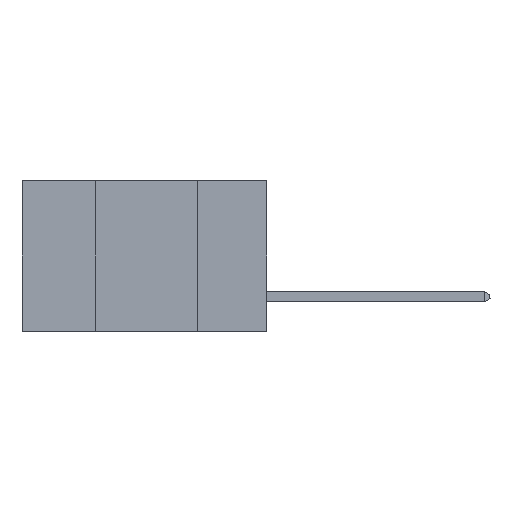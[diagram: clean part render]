
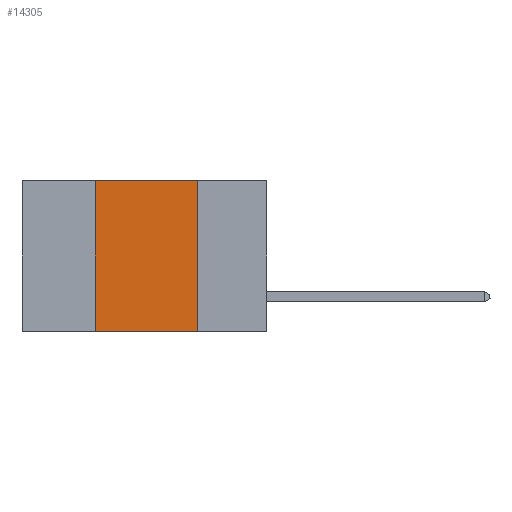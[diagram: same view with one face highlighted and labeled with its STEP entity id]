
A CAD part, left-side view. The second image highlights one B-rep face of the part: STEP entity #14305.
In plain terms, the highlighted planar face has unit normal (-1, 0, 0).
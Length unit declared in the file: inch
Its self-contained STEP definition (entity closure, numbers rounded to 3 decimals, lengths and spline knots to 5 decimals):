
#209 = VERTEX_POINT ( 'NONE', #5152 ) ;
#274 = DIRECTION ( 'NONE',  ( 0., -1., 0. ) ) ;
#516 = VECTOR ( 'NONE', #6202, 39.37008 ) ;
#661 = EDGE_CURVE ( 'NONE', #4542, #8828, #1720, .T. ) ;
#758 = CARTESIAN_POINT ( 'NONE',  ( 0., 0.6, 0. ) ) ;
#1427 = DIRECTION ( 'NONE',  ( 0., 0., 1. ) ) ;
#1720 = LINE ( 'NONE', #16820, #3463 ) ;
#3034 = VECTOR ( 'NONE', #1427, 39.37008 ) ;
#3463 = VECTOR ( 'NONE', #274, 39.37008 ) ;
#3798 = LINE ( 'NONE', #10688, #13195 ) ;
#4293 = CARTESIAN_POINT ( 'NONE',  ( 0., 0.42, 0. ) ) ;
#4542 = VERTEX_POINT ( 'NONE', #6845 ) ;
#5097 = PLANE ( 'NONE',  #12184 ) ;
#5152 = CARTESIAN_POINT ( 'NONE',  ( 0., 0.17, 0. ) ) ;
#6202 = DIRECTION ( 'NONE',  ( 0., 0., -1. ) ) ;
#6217 = EDGE_CURVE ( 'NONE', #14842, #209, #3798, .T. ) ;
#6487 = DIRECTION ( 'NONE',  ( 0., -1., 0. ) ) ;
#6845 = CARTESIAN_POINT ( 'NONE',  ( 0., 0.42, -0.37 ) ) ;
#7618 = DIRECTION ( 'NONE',  ( 1., 0., 0. ) ) ;
#7664 = FACE_OUTER_BOUND ( 'NONE', #11288, .T. ) ;
#8828 = VERTEX_POINT ( 'NONE', #13279 ) ;
#9986 = EDGE_CURVE ( 'NONE', #4542, #14842, #15908, .T. ) ;
#10352 = CARTESIAN_POINT ( 'NONE',  ( 0., 0.17, 0. ) ) ;
#10570 = ORIENTED_EDGE ( 'NONE', *, *, #9986, .F. ) ;
#10688 = CARTESIAN_POINT ( 'NONE',  ( 0., 0.6, 0. ) ) ;
#11288 = EDGE_LOOP ( 'NONE', ( #16952, #12629, #10570, #17059 ) ) ;
#12184 = AXIS2_PLACEMENT_3D ( 'NONE', #758, #7618, #13270 ) ;
#12629 = ORIENTED_EDGE ( 'NONE', *, *, #6217, .F. ) ;
#13195 = VECTOR ( 'NONE', #6487, 39.37008 ) ;
#13270 = DIRECTION ( 'NONE',  ( 0., 0., -1. ) ) ;
#13279 = CARTESIAN_POINT ( 'NONE',  ( 0., 0.17, -0.37 ) ) ;
#13339 = EDGE_CURVE ( 'NONE', #209, #8828, #14274, .T. ) ;
#14274 = LINE ( 'NONE', #10352, #516 ) ;
#14305 = ADVANCED_FACE ( 'NONE', ( #7664 ), #5097, .F. ) ;
#14534 = CARTESIAN_POINT ( 'NONE',  ( 0., 0.42, 0. ) ) ;
#14842 = VERTEX_POINT ( 'NONE', #14534 ) ;
#15908 = LINE ( 'NONE', #4293, #3034 ) ;
#16820 = CARTESIAN_POINT ( 'NONE',  ( 0., 0.6, -0.37 ) ) ;
#16952 = ORIENTED_EDGE ( 'NONE', *, *, #13339, .F. ) ;
#17059 = ORIENTED_EDGE ( 'NONE', *, *, #661, .T. ) ;
